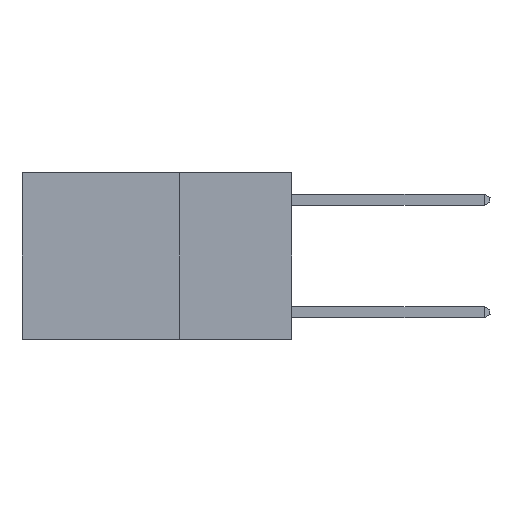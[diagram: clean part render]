
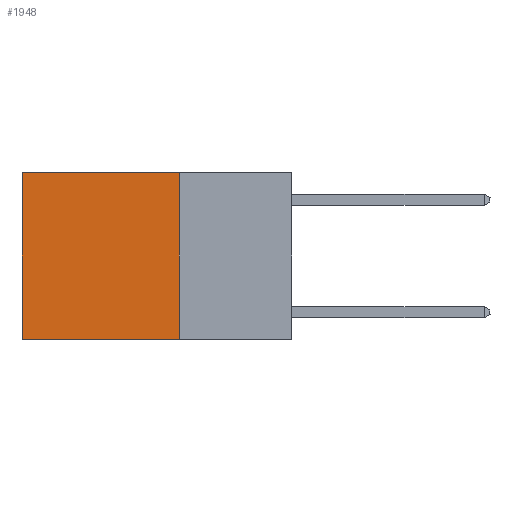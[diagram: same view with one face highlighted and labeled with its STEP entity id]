
A CAD part, left-side view. The second image highlights one B-rep face of the part: STEP entity #1948.
In plain terms, the highlighted planar face has unit normal (-1, 0, 0).
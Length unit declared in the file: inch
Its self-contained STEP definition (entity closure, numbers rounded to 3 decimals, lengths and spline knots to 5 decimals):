
#377 = CARTESIAN_POINT ( 'NONE',  ( 0.2625, 0.6, 0. ) ) ;
#429 = ORIENTED_EDGE ( 'NONE', *, *, #17291, .F. ) ;
#887 = CARTESIAN_POINT ( 'NONE',  ( 0.2625, 0.6, 0. ) ) ;
#1454 = DIRECTION ( 'NONE',  ( 0., 1., 0. ) ) ;
#1863 = LINE ( 'NONE', #887, #3046 ) ;
#1948 = ADVANCED_FACE ( 'NONE', ( #5676 ), #12923, .F. ) ;
#2403 = DIRECTION ( 'NONE',  ( 0., 0., -1. ) ) ;
#2463 = EDGE_CURVE ( 'NONE', #11228, #13233, #11624, .T. ) ;
#2788 = CARTESIAN_POINT ( 'NONE',  ( 0.2625, 0.25, 0. ) ) ;
#3046 = VECTOR ( 'NONE', #11130, 39.37008 ) ;
#3188 = VERTEX_POINT ( 'NONE', #377 ) ;
#3200 = ORIENTED_EDGE ( 'NONE', *, *, #2463, .F. ) ;
#4264 = CARTESIAN_POINT ( 'NONE',  ( 0.2625, 0.25, 0. ) ) ;
#5353 = DIRECTION ( 'NONE',  ( 0., 1., 0. ) ) ;
#5546 = VECTOR ( 'NONE', #5353, 39.37008 ) ;
#5676 = FACE_OUTER_BOUND ( 'NONE', #17622, .T. ) ;
#5798 = CARTESIAN_POINT ( 'NONE',  ( 0.2625, 0.25, 0. ) ) ;
#5894 = LINE ( 'NONE', #5798, #8239 ) ;
#8239 = VECTOR ( 'NONE', #1454, 39.37008 ) ;
#8870 = VECTOR ( 'NONE', #14332, 39.37008 ) ;
#9601 = LINE ( 'NONE', #15504, #5546 ) ;
#10578 = AXIS2_PLACEMENT_3D ( 'NONE', #2788, #17461, #2403 ) ;
#10889 = ORIENTED_EDGE ( 'NONE', *, *, #14687, .T. ) ;
#11130 = DIRECTION ( 'NONE',  ( 0., 0., -1. ) ) ;
#11228 = VERTEX_POINT ( 'NONE', #18669 ) ;
#11624 = LINE ( 'NONE', #4264, #8870 ) ;
#12923 = PLANE ( 'NONE',  #10578 ) ;
#13233 = VERTEX_POINT ( 'NONE', #13334 ) ;
#13334 = CARTESIAN_POINT ( 'NONE',  ( 0.2625, 0.25, -0.37 ) ) ;
#14332 = DIRECTION ( 'NONE',  ( 0., 0., -1. ) ) ;
#14687 = EDGE_CURVE ( 'NONE', #11228, #3188, #5894, .T. ) ;
#15504 = CARTESIAN_POINT ( 'NONE',  ( 0.2625, 0.25, -0.37 ) ) ;
#15842 = ORIENTED_EDGE ( 'NONE', *, *, #16383, .T. ) ;
#16383 = EDGE_CURVE ( 'NONE', #3188, #18727, #1863, .T. ) ;
#17291 = EDGE_CURVE ( 'NONE', #13233, #18727, #9601, .T. ) ;
#17461 = DIRECTION ( 'NONE',  ( 1., 0., 0. ) ) ;
#17622 = EDGE_LOOP ( 'NONE', ( #15842, #429, #3200, #10889 ) ) ;
#18669 = CARTESIAN_POINT ( 'NONE',  ( 0.2625, 0.25, 0. ) ) ;
#18727 = VERTEX_POINT ( 'NONE', #18787 ) ;
#18787 = CARTESIAN_POINT ( 'NONE',  ( 0.2625, 0.6, -0.37 ) ) ;
